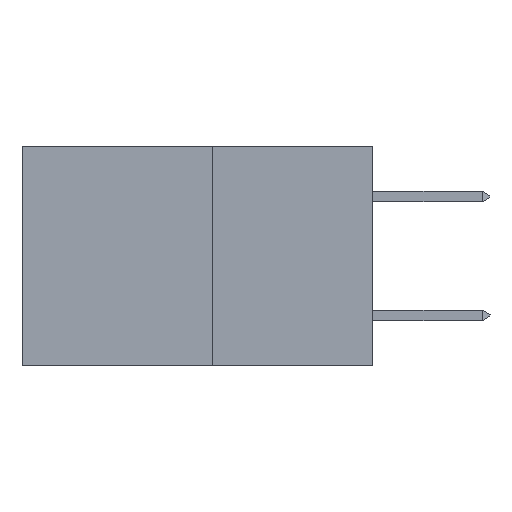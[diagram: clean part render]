
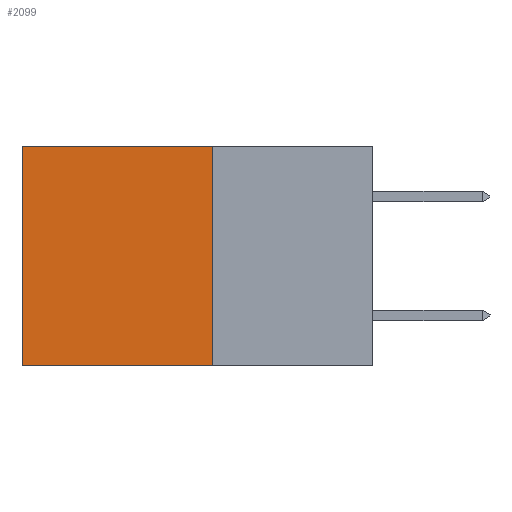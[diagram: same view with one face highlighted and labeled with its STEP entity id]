
A CAD part, left-side view. The second image highlights one B-rep face of the part: STEP entity #2099.
In plain terms, the highlighted planar face has unit normal (-1, 0, 0).
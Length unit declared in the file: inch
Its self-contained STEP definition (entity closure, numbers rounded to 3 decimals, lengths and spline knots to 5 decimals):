
#101 = CARTESIAN_POINT ( 'NONE',  ( 0.277, 0.27, -0.37 ) ) ;
#683 = ORIENTED_EDGE ( 'NONE', *, *, #4160, .T. ) ;
#1024 = CARTESIAN_POINT ( 'NONE',  ( 0.277, 0.27, 0. ) ) ;
#2099 = ADVANCED_FACE ( 'NONE', ( #9398 ), #19945, .F. ) ;
#3564 = ORIENTED_EDGE ( 'NONE', *, *, #12996, .T. ) ;
#4160 = EDGE_CURVE ( 'NONE', #18791, #16254, #4663, .T. ) ;
#4452 = VECTOR ( 'NONE', #21718, 39.37008 ) ;
#4663 = LINE ( 'NONE', #17540, #23543 ) ;
#5377 = ORIENTED_EDGE ( 'NONE', *, *, #24281, .F. ) ;
#6835 = CARTESIAN_POINT ( 'NONE',  ( 0.277, 0.59, -0.37 ) ) ;
#7586 = DIRECTION ( 'NONE',  ( 0., 0., -1. ) ) ;
#7673 = DIRECTION ( 'NONE',  ( 1., 0., 0. ) ) ;
#8142 = CARTESIAN_POINT ( 'NONE',  ( 0.277, 0.59, -0.37 ) ) ;
#9242 = DIRECTION ( 'NONE',  ( 0., 1., 0. ) ) ;
#9398 = FACE_OUTER_BOUND ( 'NONE', #23967, .T. ) ;
#9664 = LINE ( 'NONE', #19780, #4452 ) ;
#12305 = ORIENTED_EDGE ( 'NONE', *, *, #21280, .F. ) ;
#12996 = EDGE_CURVE ( 'NONE', #16254, #20832, #20272, .T. ) ;
#15022 = LINE ( 'NONE', #19010, #24625 ) ;
#16254 = VERTEX_POINT ( 'NONE', #18894 ) ;
#17540 = CARTESIAN_POINT ( 'NONE',  ( 0.277, 0.27, 0. ) ) ;
#18791 = VERTEX_POINT ( 'NONE', #1024 ) ;
#18894 = CARTESIAN_POINT ( 'NONE',  ( 0.277, 0.59, 0. ) ) ;
#19010 = CARTESIAN_POINT ( 'NONE',  ( 0.277, 0.27, -0.37 ) ) ;
#19780 = CARTESIAN_POINT ( 'NONE',  ( 0.277, 0.27, -0.37 ) ) ;
#19945 = PLANE ( 'NONE',  #25044 ) ;
#20272 = LINE ( 'NONE', #8142, #20896 ) ;
#20717 = DIRECTION ( 'NONE',  ( 0., 1., 0. ) ) ;
#20832 = VERTEX_POINT ( 'NONE', #6835 ) ;
#20896 = VECTOR ( 'NONE', #23686, 39.37008 ) ;
#21280 = EDGE_CURVE ( 'NONE', #18791, #23270, #9664, .T. ) ;
#21718 = DIRECTION ( 'NONE',  ( 0., 0., -1. ) ) ;
#23204 = CARTESIAN_POINT ( 'NONE',  ( 0.277, 0.27, -0.37 ) ) ;
#23270 = VERTEX_POINT ( 'NONE', #101 ) ;
#23543 = VECTOR ( 'NONE', #20717, 39.37008 ) ;
#23686 = DIRECTION ( 'NONE',  ( 0., 0., -1. ) ) ;
#23967 = EDGE_LOOP ( 'NONE', ( #3564, #5377, #12305, #683 ) ) ;
#24281 = EDGE_CURVE ( 'NONE', #23270, #20832, #15022, .T. ) ;
#24625 = VECTOR ( 'NONE', #9242, 39.37008 ) ;
#25044 = AXIS2_PLACEMENT_3D ( 'NONE', #23204, #7673, #7586 ) ;
